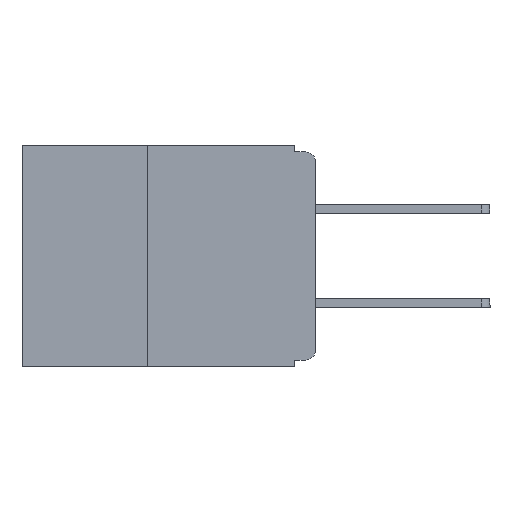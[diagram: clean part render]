
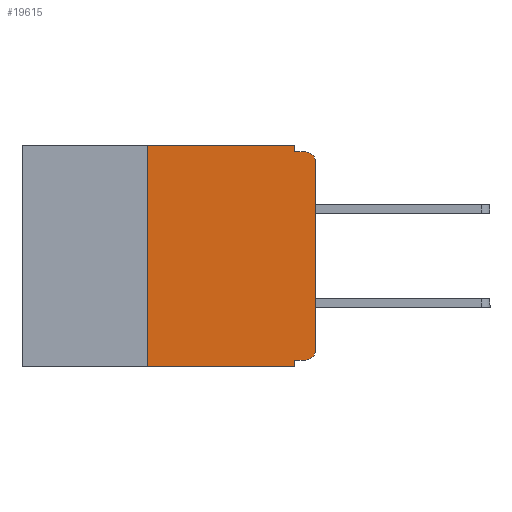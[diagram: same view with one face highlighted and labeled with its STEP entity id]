
A CAD part, left-side view. The second image highlights one B-rep face of the part: STEP entity #19615.
In plain terms, the highlighted planar face has unit normal (-1, 0, 0).
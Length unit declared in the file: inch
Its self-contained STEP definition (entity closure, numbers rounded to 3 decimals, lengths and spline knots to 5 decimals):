
#65 = CARTESIAN_POINT ( 'NONE',  ( 0., 0.437, 0. ) ) ;
#939 = DIRECTION ( 'NONE',  ( 0., -1., 0. ) ) ;
#944 = VECTOR ( 'NONE', #10024, 39.37008 ) ;
#1106 = EDGE_CURVE ( 'NONE', #25529, #12344, #1374, .T. ) ;
#1202 = VERTEX_POINT ( 'NONE', #23759 ) ;
#1374 = CIRCLE ( 'NONE', #34172, 0.015 ) ;
#1789 = CARTESIAN_POINT ( 'NONE',  ( 0., 0.031, -0.01 ) ) ;
#3410 = CARTESIAN_POINT ( 'NONE',  ( 0., 0.25, 0. ) ) ;
#3420 = EDGE_CURVE ( 'NONE', #11929, #16305, #20461, .T. ) ;
#3979 = EDGE_CURVE ( 'NONE', #11929, #31295, #18193, .T. ) ;
#5070 = AXIS2_PLACEMENT_3D ( 'NONE', #27830, #11756, #30486 ) ;
#5755 = ORIENTED_EDGE ( 'NONE', *, *, #17564, .T. ) ;
#6188 = LINE ( 'NONE', #28630, #19011 ) ;
#6316 = ORIENTED_EDGE ( 'NONE', *, *, #9244, .F. ) ;
#6427 = CARTESIAN_POINT ( 'NONE',  ( 0., 0.031, 0. ) ) ;
#7662 = DIRECTION ( 'NONE',  ( 0., 0., -1. ) ) ;
#8909 = EDGE_CURVE ( 'NONE', #26143, #33086, #22521, .T. ) ;
#9226 = VECTOR ( 'NONE', #939, 39.37008 ) ;
#9244 = EDGE_CURVE ( 'NONE', #25529, #11523, #24122, .T. ) ;
#9796 = DIRECTION ( 'NONE',  ( 0., 0., 1. ) ) ;
#9872 = CARTESIAN_POINT ( 'NONE',  ( 0., 0.031, 0. ) ) ;
#10024 = DIRECTION ( 'NONE',  ( 0., 0., -1. ) ) ;
#10195 = AXIS2_PLACEMENT_3D ( 'NONE', #21260, #23910, #7662 ) ;
#10629 = ORIENTED_EDGE ( 'NONE', *, *, #31344, .F. ) ;
#11060 = DIRECTION ( 'NONE',  ( 0., -1., 0. ) ) ;
#11382 = CARTESIAN_POINT ( 'NONE',  ( 0., 0.015, -0.32 ) ) ;
#11523 = VERTEX_POINT ( 'NONE', #33411 ) ;
#11756 = DIRECTION ( 'NONE',  ( -1., 0., 0. ) ) ;
#11929 = VERTEX_POINT ( 'NONE', #16404 ) ;
#12022 = CARTESIAN_POINT ( 'NONE',  ( 0., 0., -0.025 ) ) ;
#12217 = VECTOR ( 'NONE', #26653, 39.37008 ) ;
#12344 = VERTEX_POINT ( 'NONE', #17773 ) ;
#13558 = ORIENTED_EDGE ( 'NONE', *, *, #22951, .F. ) ;
#13742 = EDGE_CURVE ( 'NONE', #12344, #14804, #6188, .T. ) ;
#13814 = ORIENTED_EDGE ( 'NONE', *, *, #3979, .T. ) ;
#14032 = CIRCLE ( 'NONE', #5070, 0.015 ) ;
#14804 = VERTEX_POINT ( 'NONE', #12022 ) ;
#15038 = DIRECTION ( 'NONE',  ( 0., 0., 1. ) ) ;
#16305 = VERTEX_POINT ( 'NONE', #3410 ) ;
#16404 = CARTESIAN_POINT ( 'NONE',  ( 0., 0.25, -0.33 ) ) ;
#17030 = VECTOR ( 'NONE', #26716, 39.37008 ) ;
#17564 = EDGE_CURVE ( 'NONE', #14804, #1202, #14032, .T. ) ;
#17773 = CARTESIAN_POINT ( 'NONE',  ( 0., 0., -0.305 ) ) ;
#18193 = LINE ( 'NONE', #33175, #9226 ) ;
#18541 = PLANE ( 'NONE',  #10195 ) ;
#19011 = VECTOR ( 'NONE', #9796, 39.37008 ) ;
#19615 = ADVANCED_FACE ( 'NONE', ( #26056 ), #18541, .F. ) ;
#19964 = EDGE_LOOP ( 'NONE', ( #31426, #5755, #20387, #22474, #10629, #34441, #13814, #13558, #6316, #24617 ) ) ;
#19997 = LINE ( 'NONE', #26156, #944 ) ;
#20387 = ORIENTED_EDGE ( 'NONE', *, *, #30835, .F. ) ;
#20461 = LINE ( 'NONE', #31001, #28341 ) ;
#21139 = LINE ( 'NONE', #65, #12217 ) ;
#21260 = CARTESIAN_POINT ( 'NONE',  ( 0., 0.437, 0. ) ) ;
#21993 = CARTESIAN_POINT ( 'NONE',  ( 0., 0., -0.01 ) ) ;
#22474 = ORIENTED_EDGE ( 'NONE', *, *, #8909, .F. ) ;
#22521 = LINE ( 'NONE', #9872, #23347 ) ;
#22951 = EDGE_CURVE ( 'NONE', #11523, #31295, #19997, .T. ) ;
#23347 = VECTOR ( 'NONE', #26008, 39.37008 ) ;
#23670 = VECTOR ( 'NONE', #11060, 39.37008 ) ;
#23759 = CARTESIAN_POINT ( 'NONE',  ( 0., 0.015, -0.01 ) ) ;
#23910 = DIRECTION ( 'NONE',  ( 1., 0., 0. ) ) ;
#24122 = LINE ( 'NONE', #31877, #17030 ) ;
#24470 = LINE ( 'NONE', #21993, #23670 ) ;
#24617 = ORIENTED_EDGE ( 'NONE', *, *, #1106, .T. ) ;
#25529 = VERTEX_POINT ( 'NONE', #11382 ) ;
#26008 = DIRECTION ( 'NONE',  ( 0., 0., -1. ) ) ;
#26056 = FACE_OUTER_BOUND ( 'NONE', #19964, .T. ) ;
#26143 = VERTEX_POINT ( 'NONE', #6427 ) ;
#26156 = CARTESIAN_POINT ( 'NONE',  ( 0., 0.031, -0.33 ) ) ;
#26653 = DIRECTION ( 'NONE',  ( 0., -1., 0. ) ) ;
#26716 = DIRECTION ( 'NONE',  ( 0., 1., 0. ) ) ;
#27830 = CARTESIAN_POINT ( 'NONE',  ( 0., 0.015, -0.025 ) ) ;
#28341 = VECTOR ( 'NONE', #15038, 39.37008 ) ;
#28630 = CARTESIAN_POINT ( 'NONE',  ( 0., 0., 0. ) ) ;
#29347 = CARTESIAN_POINT ( 'NONE',  ( 0., 0.031, -0.33 ) ) ;
#30486 = DIRECTION ( 'NONE',  ( 0., 0., -1. ) ) ;
#30835 = EDGE_CURVE ( 'NONE', #33086, #1202, #24470, .T. ) ;
#31001 = CARTESIAN_POINT ( 'NONE',  ( 0., 0.25, -0.33 ) ) ;
#31295 = VERTEX_POINT ( 'NONE', #29347 ) ;
#31344 = EDGE_CURVE ( 'NONE', #16305, #26143, #21139, .T. ) ;
#31426 = ORIENTED_EDGE ( 'NONE', *, *, #13742, .T. ) ;
#31500 = DIRECTION ( 'NONE',  ( 0., 0., -1. ) ) ;
#31536 = DIRECTION ( 'NONE',  ( -1., 0., 0. ) ) ;
#31581 = CARTESIAN_POINT ( 'NONE',  ( 0., 0.015, -0.305 ) ) ;
#31877 = CARTESIAN_POINT ( 'NONE',  ( 0., 0., -0.32 ) ) ;
#33086 = VERTEX_POINT ( 'NONE', #1789 ) ;
#33175 = CARTESIAN_POINT ( 'NONE',  ( 0., 0.437, -0.33 ) ) ;
#33411 = CARTESIAN_POINT ( 'NONE',  ( 0., 0.031, -0.32 ) ) ;
#34172 = AXIS2_PLACEMENT_3D ( 'NONE', #31581, #31536, #31500 ) ;
#34441 = ORIENTED_EDGE ( 'NONE', *, *, #3420, .F. ) ;
